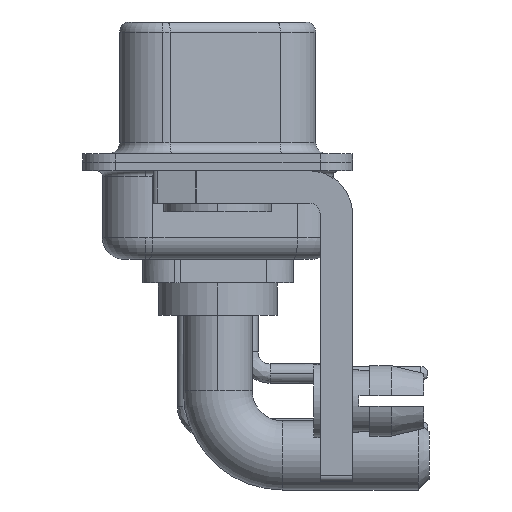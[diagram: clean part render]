
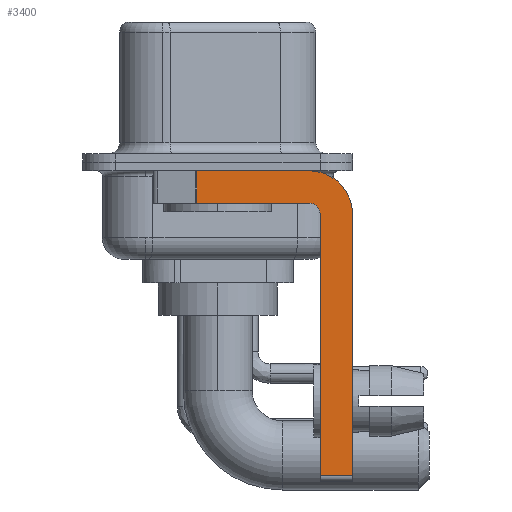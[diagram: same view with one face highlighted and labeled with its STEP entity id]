
A CAD part, left-side view. The second image highlights one B-rep face of the part: STEP entity #3400.
In plain terms, the highlighted planar face has unit normal (-1, 0, 0).
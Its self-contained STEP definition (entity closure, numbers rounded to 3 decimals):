
#18 = AXIS2_PLACEMENT_3D ( 'NONE', #17364, #25327, #23426 ) ;
#446 = CIRCLE ( 'NONE', #18, 2. ) ;
#920 = CARTESIAN_POINT ( 'NONE',  ( -2.9, 3., -0.4 ) ) ;
#960 = LINE ( 'NONE', #3145, #21450 ) ;
#1127 = ORIENTED_EDGE ( 'NONE', *, *, #9049, .F. ) ;
#1193 = CARTESIAN_POINT ( 'NONE',  ( -2.9, -4.75, -14.55 ) ) ;
#3145 = CARTESIAN_POINT ( 'NONE',  ( -2.9, -6.25, -2.4 ) ) ;
#3400 = ADVANCED_FACE ( 'NONE', ( #25057 ), #14621, .F. ) ;
#3565 = CARTESIAN_POINT ( 'NONE',  ( -2.9, -6.25, -2.4 ) ) ;
#3979 = EDGE_CURVE ( 'NONE', #11181, #5459, #7239, .T. ) ;
#4099 = VERTEX_POINT ( 'NONE', #1193 ) ;
#4163 = ORIENTED_EDGE ( 'NONE', *, *, #16947, .F. ) ;
#4308 = DIRECTION ( 'NONE',  ( -1., 0., 0. ) ) ;
#4456 = CARTESIAN_POINT ( 'NONE',  ( -2.9, -4.75, -14.8 ) ) ;
#4868 = VECTOR ( 'NONE', #9032, 1000. ) ;
#5072 = DIRECTION ( 'NONE',  ( 0., 0., -1. ) ) ;
#5459 = VERTEX_POINT ( 'NONE', #7824 ) ;
#5709 = CIRCLE ( 'NONE', #10122, 0.5 ) ;
#5787 = VERTEX_POINT ( 'NONE', #21261 ) ;
#6047 = VERTEX_POINT ( 'NONE', #17207 ) ;
#6150 = DIRECTION ( 'NONE',  ( 0., 1., 0. ) ) ;
#6503 = DIRECTION ( 'NONE',  ( 0., 0., 1. ) ) ;
#6603 = ORIENTED_EDGE ( 'NONE', *, *, #22078, .T. ) ;
#6912 = CARTESIAN_POINT ( 'NONE',  ( -2.9, -4.25, -2.4 ) ) ;
#7239 = LINE ( 'NONE', #920, #4868 ) ;
#7648 = ORIENTED_EDGE ( 'NONE', *, *, #3979, .F. ) ;
#7824 = CARTESIAN_POINT ( 'NONE',  ( -2.9, -4.25, -0.4 ) ) ;
#8847 = DIRECTION ( 'NONE',  ( 1., 0., 0. ) ) ;
#8884 = ORIENTED_EDGE ( 'NONE', *, *, #22312, .F. ) ;
#9032 = DIRECTION ( 'NONE',  ( 0., -1., 0. ) ) ;
#9049 = EDGE_CURVE ( 'NONE', #5787, #6047, #10547, .T. ) ;
#9852 = CARTESIAN_POINT ( 'NONE',  ( -2.9, -4.25, -14.55 ) ) ;
#10122 = AXIS2_PLACEMENT_3D ( 'NONE', #6912, #4308, #6503 ) ;
#10150 = LINE ( 'NONE', #4456, #23504 ) ;
#10487 = EDGE_CURVE ( 'NONE', #11181, #6047, #19078, .T. ) ;
#10547 = LINE ( 'NONE', #25085, #22740 ) ;
#10726 = EDGE_CURVE ( 'NONE', #4099, #21624, #10150, .T. ) ;
#10779 = DIRECTION ( 'NONE',  ( 0., 0., 1. ) ) ;
#11181 = VERTEX_POINT ( 'NONE', #16909 ) ;
#13923 = ORIENTED_EDGE ( 'NONE', *, *, #10726, .F. ) ;
#14494 = DIRECTION ( 'NONE',  ( 0., -1., 0. ) ) ;
#14621 = PLANE ( 'NONE',  #20596 ) ;
#15917 = EDGE_CURVE ( 'NONE', #25623, #16733, #960, .T. ) ;
#16733 = VERTEX_POINT ( 'NONE', #17765 ) ;
#16909 = CARTESIAN_POINT ( 'NONE',  ( -2.9, 0.978, -0.4 ) ) ;
#16947 = EDGE_CURVE ( 'NONE', #21624, #5787, #5709, .T. ) ;
#17207 = CARTESIAN_POINT ( 'NONE',  ( -2.9, 0.978, -1.9 ) ) ;
#17364 = CARTESIAN_POINT ( 'NONE',  ( -2.9, -4.25, -2.4 ) ) ;
#17765 = CARTESIAN_POINT ( 'NONE',  ( -2.9, -6.25, -14.55 ) ) ;
#19078 = LINE ( 'NONE', #21690, #21721 ) ;
#19617 = DIRECTION ( 'NONE',  ( 0., 0., -1. ) ) ;
#20280 = LINE ( 'NONE', #9852, #23688 ) ;
#20449 = CARTESIAN_POINT ( 'NONE',  ( -2.9, -4.75, -2.4 ) ) ;
#20596 = AXIS2_PLACEMENT_3D ( 'NONE', #23008, #8847, #21479 ) ;
#21261 = CARTESIAN_POINT ( 'NONE',  ( -2.9, -4.25, -1.9 ) ) ;
#21450 = VECTOR ( 'NONE', #5072, 1000. ) ;
#21479 = DIRECTION ( 'NONE',  ( 0., 0., -1. ) ) ;
#21611 = ORIENTED_EDGE ( 'NONE', *, *, #15917, .F. ) ;
#21624 = VERTEX_POINT ( 'NONE', #20449 ) ;
#21690 = CARTESIAN_POINT ( 'NONE',  ( -2.9, 0.978, -1.9 ) ) ;
#21721 = VECTOR ( 'NONE', #19617, 1000. ) ;
#22078 = EDGE_CURVE ( 'NONE', #4099, #16733, #20280, .T. ) ;
#22312 = EDGE_CURVE ( 'NONE', #5459, #25623, #446, .T. ) ;
#22740 = VECTOR ( 'NONE', #6150, 1000. ) ;
#23008 = CARTESIAN_POINT ( 'NONE',  ( -2.9, -4.25, -2.4 ) ) ;
#23426 = DIRECTION ( 'NONE',  ( 0., 0., -1. ) ) ;
#23504 = VECTOR ( 'NONE', #10779, 1000. ) ;
#23688 = VECTOR ( 'NONE', #14494, 1000. ) ;
#25057 = FACE_OUTER_BOUND ( 'NONE', #26406, .T. ) ;
#25085 = CARTESIAN_POINT ( 'NONE',  ( -2.9, -4.25, -1.9 ) ) ;
#25327 = DIRECTION ( 'NONE',  ( 1., 0., 0. ) ) ;
#25623 = VERTEX_POINT ( 'NONE', #3565 ) ;
#26406 = EDGE_LOOP ( 'NONE', ( #7648, #26492, #1127, #4163, #13923, #6603, #21611, #8884 ) ) ;
#26492 = ORIENTED_EDGE ( 'NONE', *, *, #10487, .T. ) ;
